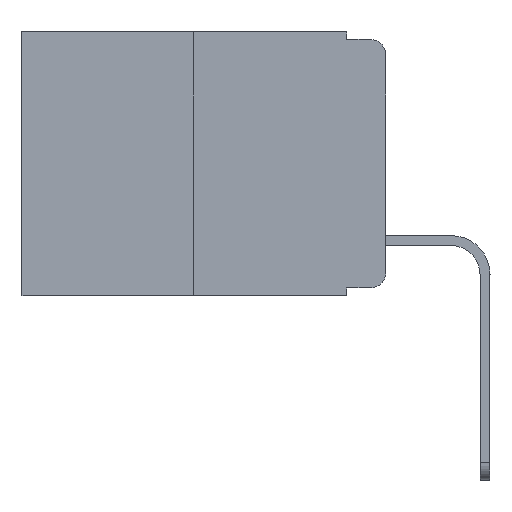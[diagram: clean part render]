
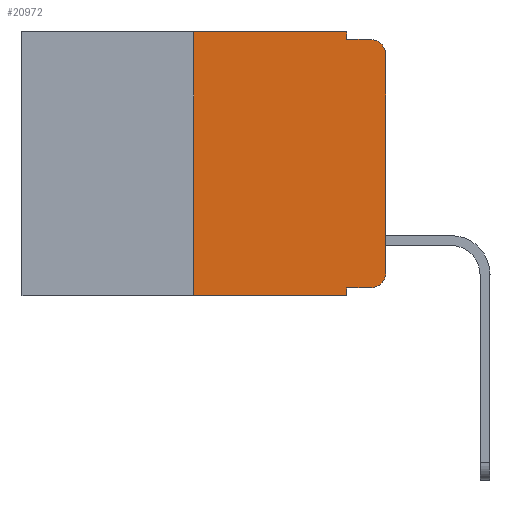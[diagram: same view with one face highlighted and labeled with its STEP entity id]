
A CAD part, left-side view. The second image highlights one B-rep face of the part: STEP entity #20972.
In plain terms, the highlighted planar face has unit normal (-1, 0, 0).
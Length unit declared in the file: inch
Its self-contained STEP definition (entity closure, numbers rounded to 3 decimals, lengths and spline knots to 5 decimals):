
#17 = CARTESIAN_POINT ( 'NONE',  ( 0., 0.051, -0.333 ) ) ;
#535 = CARTESIAN_POINT ( 'NONE',  ( 0., 0.051, -0.343 ) ) ;
#1218 = DIRECTION ( 'NONE',  ( 0., 0., 1. ) ) ;
#1275 = LINE ( 'NONE', #6002, #16562 ) ;
#1513 = DIRECTION ( 'NONE',  ( -1., 0., 0. ) ) ;
#1672 = VERTEX_POINT ( 'NONE', #21138 ) ;
#2056 = DIRECTION ( 'NONE',  ( 0., -1., 0. ) ) ;
#2196 = DIRECTION ( 'NONE',  ( 0., -1., 0. ) ) ;
#2322 = CARTESIAN_POINT ( 'NONE',  ( 0., 0.051, -0.01 ) ) ;
#2327 = VECTOR ( 'NONE', #1218, 39.37008 ) ;
#2508 = VERTEX_POINT ( 'NONE', #3480 ) ;
#2914 = LINE ( 'NONE', #8581, #20577 ) ;
#2959 = EDGE_CURVE ( 'NONE', #5324, #17340, #18966, .T. ) ;
#3399 = LINE ( 'NONE', #21778, #2327 ) ;
#3480 = CARTESIAN_POINT ( 'NONE',  ( 0., 0.051, 0. ) ) ;
#3822 = LINE ( 'NONE', #11998, #5682 ) ;
#4430 = AXIS2_PLACEMENT_3D ( 'NONE', #15079, #16654, #6332 ) ;
#4523 = CARTESIAN_POINT ( 'NONE',  ( 0., 0.02, -0.01 ) ) ;
#4787 = ORIENTED_EDGE ( 'NONE', *, *, #2959, .T. ) ;
#5324 = VERTEX_POINT ( 'NONE', #16761 ) ;
#5348 = CARTESIAN_POINT ( 'NONE',  ( 0., 0.02, -0.333 ) ) ;
#5562 = ORIENTED_EDGE ( 'NONE', *, *, #21069, .T. ) ;
#5682 = VECTOR ( 'NONE', #22140, 39.37008 ) ;
#6002 = CARTESIAN_POINT ( 'NONE',  ( 0., 0.051, 0. ) ) ;
#6221 = VERTEX_POINT ( 'NONE', #4523 ) ;
#6332 = DIRECTION ( 'NONE',  ( 0., 0., -1. ) ) ;
#6548 = PLANE ( 'NONE',  #4430 ) ;
#6694 = DIRECTION ( 'NONE',  ( 0., 0., -1. ) ) ;
#6704 = AXIS2_PLACEMENT_3D ( 'NONE', #18812, #1513, #6694 ) ;
#6896 = ORIENTED_EDGE ( 'NONE', *, *, #15037, .T. ) ;
#6980 = DIRECTION ( 'NONE',  ( 0., 0., -1. ) ) ;
#7182 = EDGE_CURVE ( 'NONE', #1672, #2508, #3822, .T. ) ;
#7460 = ORIENTED_EDGE ( 'NONE', *, *, #10208, .F. ) ;
#8215 = EDGE_CURVE ( 'NONE', #10275, #20800, #16512, .T. ) ;
#8235 = EDGE_LOOP ( 'NONE', ( #6896, #5562, #9333, #9983, #12809, #20730, #4787, #7460, #9956, #14873 ) ) ;
#8246 = EDGE_CURVE ( 'NONE', #20674, #6221, #12597, .T. ) ;
#8571 = DIRECTION ( 'NONE',  ( 0., 0., 1. ) ) ;
#8581 = CARTESIAN_POINT ( 'NONE',  ( 0., 0.051, 0. ) ) ;
#8840 = VECTOR ( 'NONE', #2196, 39.37008 ) ;
#8980 = CARTESIAN_POINT ( 'NONE',  ( 0., 0.051, -0.01 ) ) ;
#8981 = VECTOR ( 'NONE', #8571, 39.37008 ) ;
#9053 = DIRECTION ( 'NONE',  ( 0., 0., -1. ) ) ;
#9333 = ORIENTED_EDGE ( 'NONE', *, *, #8246, .F. ) ;
#9485 = FACE_OUTER_BOUND ( 'NONE', #8235, .T. ) ;
#9956 = ORIENTED_EDGE ( 'NONE', *, *, #12905, .T. ) ;
#9983 = ORIENTED_EDGE ( 'NONE', *, *, #18519, .F. ) ;
#10146 = CARTESIAN_POINT ( 'NONE',  ( 0., 0.25, 0. ) ) ;
#10208 = EDGE_CURVE ( 'NONE', #13047, #17340, #2914, .T. ) ;
#10275 = VERTEX_POINT ( 'NONE', #5348 ) ;
#10464 = DIRECTION ( 'NONE',  ( -1., 0., 0. ) ) ;
#11976 = DIRECTION ( 'NONE',  ( 0., -1., 0. ) ) ;
#11998 = CARTESIAN_POINT ( 'NONE',  ( 0., 0.473, 0. ) ) ;
#12262 = CARTESIAN_POINT ( 'NONE',  ( 0., 0.473, -0.343 ) ) ;
#12597 = LINE ( 'NONE', #8980, #8840 ) ;
#12809 = ORIENTED_EDGE ( 'NONE', *, *, #7182, .F. ) ;
#12905 = EDGE_CURVE ( 'NONE', #13047, #10275, #22031, .T. ) ;
#13047 = VERTEX_POINT ( 'NONE', #16098 ) ;
#14094 = CARTESIAN_POINT ( 'NONE',  ( 0., 0., -0.03 ) ) ;
#14128 = VECTOR ( 'NONE', #2056, 39.37008 ) ;
#14321 = VECTOR ( 'NONE', #11976, 39.37008 ) ;
#14873 = ORIENTED_EDGE ( 'NONE', *, *, #8215, .T. ) ;
#15037 = EDGE_CURVE ( 'NONE', #20800, #22070, #3399, .T. ) ;
#15079 = CARTESIAN_POINT ( 'NONE',  ( 0., 0.473, 0. ) ) ;
#15492 = EDGE_CURVE ( 'NONE', #5324, #1672, #18093, .T. ) ;
#15626 = AXIS2_PLACEMENT_3D ( 'NONE', #20722, #10464, #9053 ) ;
#16098 = CARTESIAN_POINT ( 'NONE',  ( 0., 0.051, -0.333 ) ) ;
#16512 = CIRCLE ( 'NONE', #15626, 0.02 ) ;
#16562 = VECTOR ( 'NONE', #17982, 39.37008 ) ;
#16654 = DIRECTION ( 'NONE',  ( 1., 0., 0. ) ) ;
#16761 = CARTESIAN_POINT ( 'NONE',  ( 0., 0.25, -0.343 ) ) ;
#17340 = VERTEX_POINT ( 'NONE', #535 ) ;
#17982 = DIRECTION ( 'NONE',  ( 0., 0., -1. ) ) ;
#18093 = LINE ( 'NONE', #10146, #8981 ) ;
#18519 = EDGE_CURVE ( 'NONE', #2508, #20674, #1275, .T. ) ;
#18812 = CARTESIAN_POINT ( 'NONE',  ( 0., 0.02, -0.03 ) ) ;
#18966 = LINE ( 'NONE', #12262, #14128 ) ;
#19305 = CARTESIAN_POINT ( 'NONE',  ( 0., 0., -0.313 ) ) ;
#20577 = VECTOR ( 'NONE', #6980, 39.37008 ) ;
#20674 = VERTEX_POINT ( 'NONE', #2322 ) ;
#20722 = CARTESIAN_POINT ( 'NONE',  ( 0., 0.02, -0.313 ) ) ;
#20730 = ORIENTED_EDGE ( 'NONE', *, *, #15492, .F. ) ;
#20800 = VERTEX_POINT ( 'NONE', #19305 ) ;
#20972 = ADVANCED_FACE ( 'NONE', ( #9485 ), #6548, .F. ) ;
#21069 = EDGE_CURVE ( 'NONE', #22070, #6221, #21270, .T. ) ;
#21138 = CARTESIAN_POINT ( 'NONE',  ( 0., 0.25, 0. ) ) ;
#21270 = CIRCLE ( 'NONE', #6704, 0.02 ) ;
#21778 = CARTESIAN_POINT ( 'NONE',  ( 0., 0., 0. ) ) ;
#22031 = LINE ( 'NONE', #17, #14321 ) ;
#22070 = VERTEX_POINT ( 'NONE', #14094 ) ;
#22140 = DIRECTION ( 'NONE',  ( 0., -1., 0. ) ) ;
